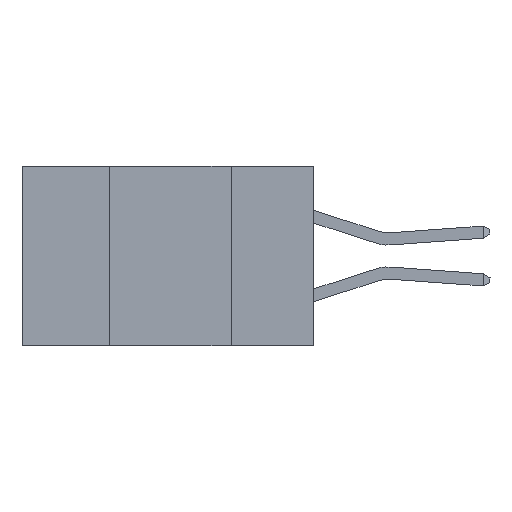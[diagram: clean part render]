
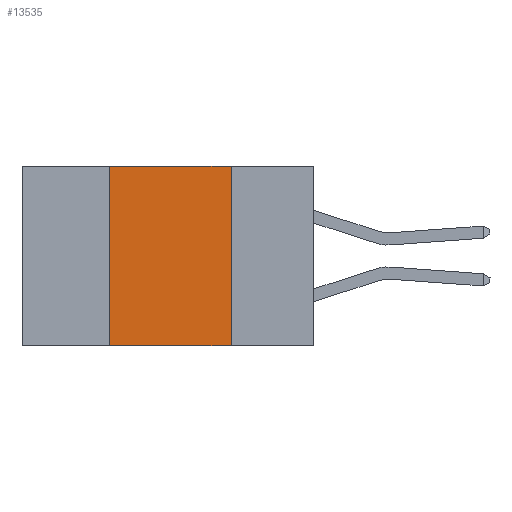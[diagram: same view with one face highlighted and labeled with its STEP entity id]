
A CAD part, left-side view. The second image highlights one B-rep face of the part: STEP entity #13535.
In plain terms, the highlighted planar face has unit normal (-1, 0, 0).
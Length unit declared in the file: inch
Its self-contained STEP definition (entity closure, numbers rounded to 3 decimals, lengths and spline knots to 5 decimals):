
#613 = VERTEX_POINT ( 'NONE', #23083 ) ;
#680 = CARTESIAN_POINT ( 'NONE',  ( 0., 0.6, -0.37 ) ) ;
#1195 = EDGE_CURVE ( 'NONE', #613, #3251, #3107, .T. ) ;
#1885 = CARTESIAN_POINT ( 'NONE',  ( 0., 0.42, 0. ) ) ;
#3107 = LINE ( 'NONE', #21574, #5949 ) ;
#3251 = VERTEX_POINT ( 'NONE', #3555 ) ;
#3521 = CARTESIAN_POINT ( 'NONE',  ( 0., 0.42, -0.37 ) ) ;
#3555 = CARTESIAN_POINT ( 'NONE',  ( 0., 0.17, 0. ) ) ;
#3712 = VERTEX_POINT ( 'NONE', #3521 ) ;
#4615 = AXIS2_PLACEMENT_3D ( 'NONE', #13707, #21164, #20921 ) ;
#4689 = VECTOR ( 'NONE', #11933, 39.37008 ) ;
#4757 = FACE_OUTER_BOUND ( 'NONE', #5598, .T. ) ;
#5598 = EDGE_LOOP ( 'NONE', ( #22607, #14555, #11650, #18454 ) ) ;
#5949 = VECTOR ( 'NONE', #14481, 39.37008 ) ;
#6348 = PLANE ( 'NONE',  #4615 ) ;
#7113 = CARTESIAN_POINT ( 'NONE',  ( 0., 0.17, 0. ) ) ;
#8078 = DIRECTION ( 'NONE',  ( 0., -1., 0. ) ) ;
#10384 = EDGE_CURVE ( 'NONE', #3251, #17951, #16285, .T. ) ;
#11650 = ORIENTED_EDGE ( 'NONE', *, *, #15715, .F. ) ;
#11702 = LINE ( 'NONE', #680, #17374 ) ;
#11933 = DIRECTION ( 'NONE',  ( 0., 0., 1. ) ) ;
#12918 = LINE ( 'NONE', #1885, #4689 ) ;
#13535 = ADVANCED_FACE ( 'NONE', ( #4757 ), #6348, .F. ) ;
#13707 = CARTESIAN_POINT ( 'NONE',  ( 0., 0.6, 0. ) ) ;
#13799 = CARTESIAN_POINT ( 'NONE',  ( 0., 0.17, -0.37 ) ) ;
#14475 = DIRECTION ( 'NONE',  ( 0., 0., -1. ) ) ;
#14481 = DIRECTION ( 'NONE',  ( 0., -1., 0. ) ) ;
#14555 = ORIENTED_EDGE ( 'NONE', *, *, #1195, .F. ) ;
#15715 = EDGE_CURVE ( 'NONE', #3712, #613, #12918, .T. ) ;
#16285 = LINE ( 'NONE', #7113, #16895 ) ;
#16895 = VECTOR ( 'NONE', #14475, 39.37008 ) ;
#17013 = EDGE_CURVE ( 'NONE', #3712, #17951, #11702, .T. ) ;
#17374 = VECTOR ( 'NONE', #8078, 39.37008 ) ;
#17951 = VERTEX_POINT ( 'NONE', #13799 ) ;
#18454 = ORIENTED_EDGE ( 'NONE', *, *, #17013, .T. ) ;
#20921 = DIRECTION ( 'NONE',  ( 0., 0., -1. ) ) ;
#21164 = DIRECTION ( 'NONE',  ( 1., 0., 0. ) ) ;
#21574 = CARTESIAN_POINT ( 'NONE',  ( 0., 0.6, 0. ) ) ;
#22607 = ORIENTED_EDGE ( 'NONE', *, *, #10384, .F. ) ;
#23083 = CARTESIAN_POINT ( 'NONE',  ( 0., 0.42, 0. ) ) ;
